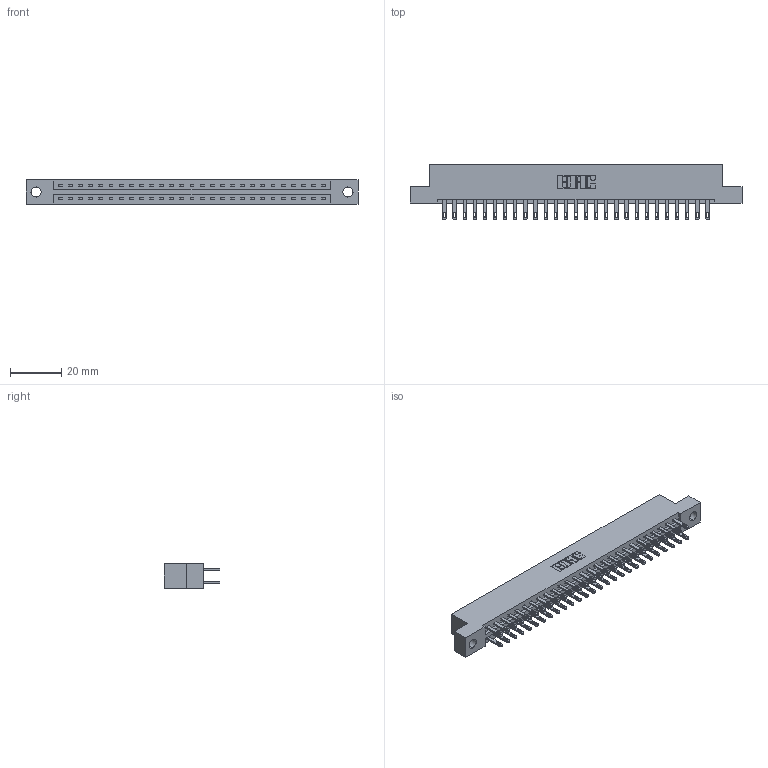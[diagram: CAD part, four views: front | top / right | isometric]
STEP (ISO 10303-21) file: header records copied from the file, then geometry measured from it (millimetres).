
FILE_DESCRIPTION (( 'STEP AP203' ), '1' );
FILE_NAME ('887-054-500-204.STEP', '2020-09-21T01:28:51', ( '' ), ( '' ), 'SwSTEP 2.0', 'SolidWorks 2020', '' );
FILE_SCHEMA (( 'CONFIG_CONTROL_DESIGN' ));
Length unit declared in the file: inch
Products named in the file (3): 345-292-001_345-293-100; 887-054-500-204; 837 Part_Flush Mounting Lugs - 0.156 Dia-TH
Assembly tree (55 placements, depth 2):
  887-054-500-204
    837 Part_Flush Mounting Lugs - 0.156 Dia-TH
    345-292-001_345-293-100  x54
Bounding box: 130 x 21.85 x 9.4 mm (x, y, z)
Volume: 13577.6 mm3; surface area: 15600.4 mm2
Topology: 55 solids, 55 shells, 2814 faces, 8573 edges, 5714 vertices
Faces by surface type: plane 1798, cylinder 1016
Entity records: 22807 total; most frequent: CARTESIAN_POINT 3854, ORIENTED_EDGE 3790, DIRECTION 3307, EDGE_CURVE 1895, LINE 1763, VECTOR 1763, VERTEX_POINT 1262, AXIS2_PLACEMENT_3D 772
